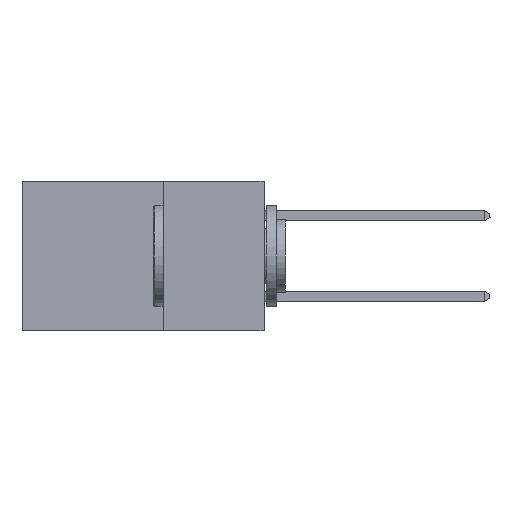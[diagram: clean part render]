
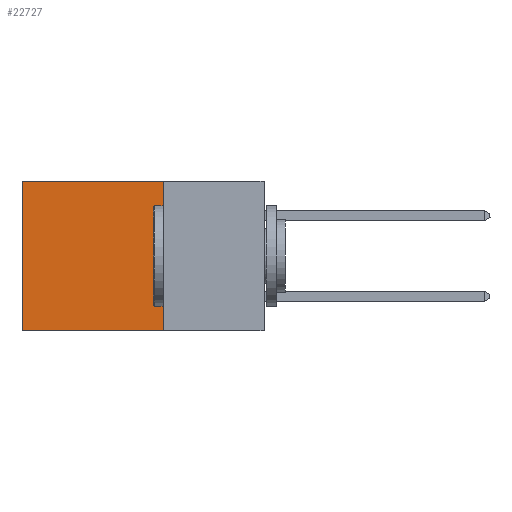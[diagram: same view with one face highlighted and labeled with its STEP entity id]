
A CAD part, left-side view. The second image highlights one B-rep face of the part: STEP entity #22727.
In plain terms, the highlighted planar face has unit normal (-1, 0, 0).
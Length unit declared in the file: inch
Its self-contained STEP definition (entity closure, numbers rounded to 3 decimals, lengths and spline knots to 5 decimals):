
#83 = EDGE_LOOP ( 'NONE', ( #9469, #16491, #15501, #25231 ) ) ;
#107 = EDGE_CURVE ( 'NONE', #12999, #17036, #6173, .T. ) ;
#164 = VECTOR ( 'NONE', #14250, 39.37008 ) ;
#338 = DIRECTION ( 'NONE',  ( 0., 0., -1. ) ) ;
#2713 = CARTESIAN_POINT ( 'NONE',  ( 0.298, 0.6, -0.37 ) ) ;
#3464 = EDGE_CURVE ( 'NONE', #6276, #17036, #14520, .T. ) ;
#4446 = CARTESIAN_POINT ( 'NONE',  ( 0.298, 0.25, 0. ) ) ;
#5378 = CARTESIAN_POINT ( 'NONE',  ( 0.298, 0.6, 0. ) ) ;
#5875 = LINE ( 'NONE', #4446, #20416 ) ;
#6173 = LINE ( 'NONE', #24383, #164 ) ;
#6276 = VERTEX_POINT ( 'NONE', #7100 ) ;
#7100 = CARTESIAN_POINT ( 'NONE',  ( 0.298, 0.25, -0.37 ) ) ;
#9469 = ORIENTED_EDGE ( 'NONE', *, *, #107, .T. ) ;
#10825 = AXIS2_PLACEMENT_3D ( 'NONE', #12532, #12442, #338 ) ;
#11630 = CARTESIAN_POINT ( 'NONE',  ( 0.298, 0.25, -0.37 ) ) ;
#12442 = DIRECTION ( 'NONE',  ( 1., 0., 0. ) ) ;
#12532 = CARTESIAN_POINT ( 'NONE',  ( 0.298, 0.25, 0. ) ) ;
#12999 = VERTEX_POINT ( 'NONE', #5378 ) ;
#13652 = LINE ( 'NONE', #22139, #25039 ) ;
#14250 = DIRECTION ( 'NONE',  ( 0., 0., -1. ) ) ;
#14520 = LINE ( 'NONE', #11630, #18931 ) ;
#15501 = ORIENTED_EDGE ( 'NONE', *, *, #25362, .F. ) ;
#16491 = ORIENTED_EDGE ( 'NONE', *, *, #3464, .F. ) ;
#16507 = DIRECTION ( 'NONE',  ( 0., 1., 0. ) ) ;
#17036 = VERTEX_POINT ( 'NONE', #2713 ) ;
#17501 = EDGE_CURVE ( 'NONE', #20969, #12999, #5875, .T. ) ;
#17583 = DIRECTION ( 'NONE',  ( 0., 1., 0. ) ) ;
#17623 = FACE_OUTER_BOUND ( 'NONE', #83, .T. ) ;
#18931 = VECTOR ( 'NONE', #17583, 39.37008 ) ;
#19879 = DIRECTION ( 'NONE',  ( 0., 0., -1. ) ) ;
#20416 = VECTOR ( 'NONE', #16507, 39.37008 ) ;
#20852 = CARTESIAN_POINT ( 'NONE',  ( 0.298, 0.25, 0. ) ) ;
#20969 = VERTEX_POINT ( 'NONE', #20852 ) ;
#22139 = CARTESIAN_POINT ( 'NONE',  ( 0.298, 0.25, 0. ) ) ;
#22727 = ADVANCED_FACE ( 'NONE', ( #17623 ), #24523, .F. ) ;
#24383 = CARTESIAN_POINT ( 'NONE',  ( 0.298, 0.6, 0. ) ) ;
#24523 = PLANE ( 'NONE',  #10825 ) ;
#25039 = VECTOR ( 'NONE', #19879, 39.37008 ) ;
#25231 = ORIENTED_EDGE ( 'NONE', *, *, #17501, .T. ) ;
#25362 = EDGE_CURVE ( 'NONE', #20969, #6276, #13652, .T. ) ;
